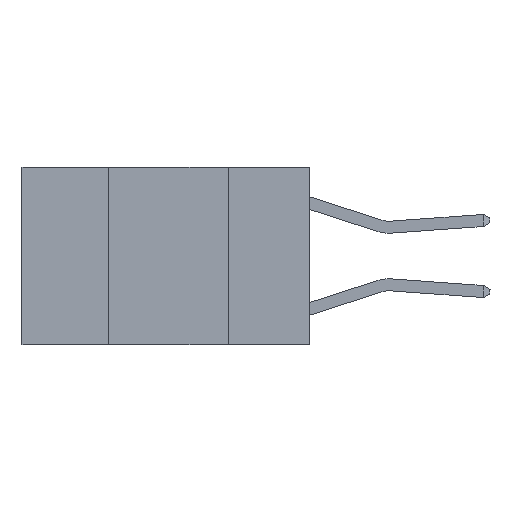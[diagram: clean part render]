
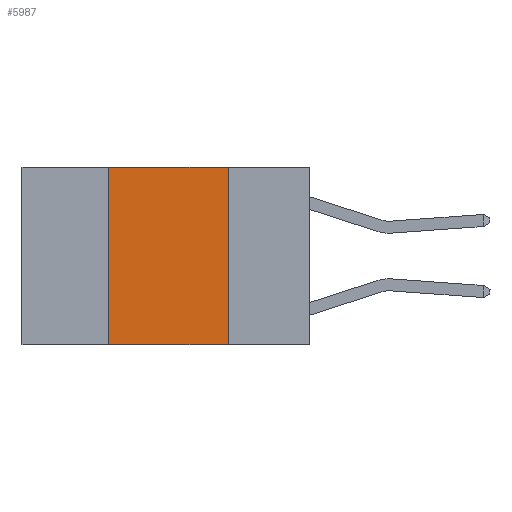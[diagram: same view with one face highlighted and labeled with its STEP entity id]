
A CAD part, left-side view. The second image highlights one B-rep face of the part: STEP entity #5987.
In plain terms, the highlighted planar face has unit normal (-1, 0, 0).
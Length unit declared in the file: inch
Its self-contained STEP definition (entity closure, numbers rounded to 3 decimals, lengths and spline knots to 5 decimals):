
#262 = CARTESIAN_POINT ( 'NONE',  ( 0., 0.17, 0. ) ) ;
#264 = VECTOR ( 'NONE', #1159, 39.37008 ) ;
#633 = LINE ( 'NONE', #4440, #1699 ) ;
#938 = CARTESIAN_POINT ( 'NONE',  ( 0., 0.42, 0. ) ) ;
#1159 = DIRECTION ( 'NONE',  ( 0., 0., 1. ) ) ;
#1471 = VECTOR ( 'NONE', #4942, 39.37008 ) ;
#1699 = VECTOR ( 'NONE', #6681, 39.37008 ) ;
#2036 = CARTESIAN_POINT ( 'NONE',  ( 0., 0.17, 0. ) ) ;
#2221 = AXIS2_PLACEMENT_3D ( 'NONE', #2625, #6187, #7855 ) ;
#2625 = CARTESIAN_POINT ( 'NONE',  ( 0., 0.6, 0. ) ) ;
#3038 = CARTESIAN_POINT ( 'NONE',  ( 0., 0.42, 0. ) ) ;
#3088 = EDGE_CURVE ( 'NONE', #4763, #5053, #633, .T. ) ;
#3101 = CARTESIAN_POINT ( 'NONE',  ( 0., 0.17, -0.37 ) ) ;
#3389 = CARTESIAN_POINT ( 'NONE',  ( 0., 0.42, -0.37 ) ) ;
#3431 = EDGE_LOOP ( 'NONE', ( #5870, #5414, #5346, #8508 ) ) ;
#3760 = LINE ( 'NONE', #3038, #264 ) ;
#3999 = FACE_OUTER_BOUND ( 'NONE', #3431, .T. ) ;
#4440 = CARTESIAN_POINT ( 'NONE',  ( 0., 0.6, -0.37 ) ) ;
#4692 = VECTOR ( 'NONE', #8003, 39.37008 ) ;
#4763 = VERTEX_POINT ( 'NONE', #3389 ) ;
#4942 = DIRECTION ( 'NONE',  ( 0., 0., -1. ) ) ;
#5053 = VERTEX_POINT ( 'NONE', #3101 ) ;
#5090 = LINE ( 'NONE', #8809, #4692 ) ;
#5185 = EDGE_CURVE ( 'NONE', #5531, #5053, #8562, .T. ) ;
#5346 = ORIENTED_EDGE ( 'NONE', *, *, #7991, .F. ) ;
#5414 = ORIENTED_EDGE ( 'NONE', *, *, #9084, .F. ) ;
#5531 = VERTEX_POINT ( 'NONE', #262 ) ;
#5870 = ORIENTED_EDGE ( 'NONE', *, *, #5185, .F. ) ;
#5987 = ADVANCED_FACE ( 'NONE', ( #3999 ), #6517, .F. ) ;
#6187 = DIRECTION ( 'NONE',  ( 1., 0., 0. ) ) ;
#6517 = PLANE ( 'NONE',  #2221 ) ;
#6681 = DIRECTION ( 'NONE',  ( 0., -1., 0. ) ) ;
#7855 = DIRECTION ( 'NONE',  ( 0., 0., -1. ) ) ;
#7991 = EDGE_CURVE ( 'NONE', #4763, #9156, #3760, .T. ) ;
#8003 = DIRECTION ( 'NONE',  ( 0., -1., 0. ) ) ;
#8508 = ORIENTED_EDGE ( 'NONE', *, *, #3088, .T. ) ;
#8562 = LINE ( 'NONE', #2036, #1471 ) ;
#8809 = CARTESIAN_POINT ( 'NONE',  ( 0., 0.6, 0. ) ) ;
#9084 = EDGE_CURVE ( 'NONE', #9156, #5531, #5090, .T. ) ;
#9156 = VERTEX_POINT ( 'NONE', #938 ) ;
